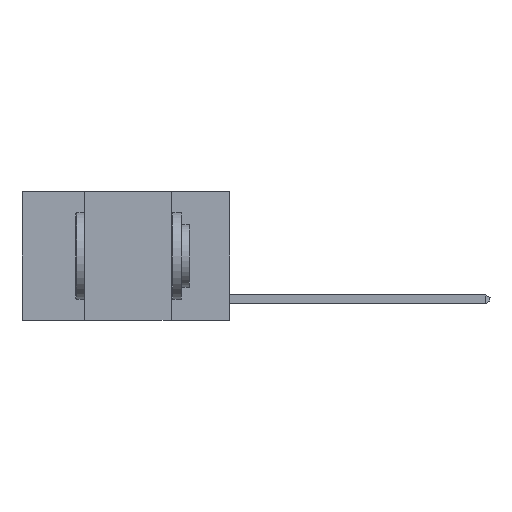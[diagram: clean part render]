
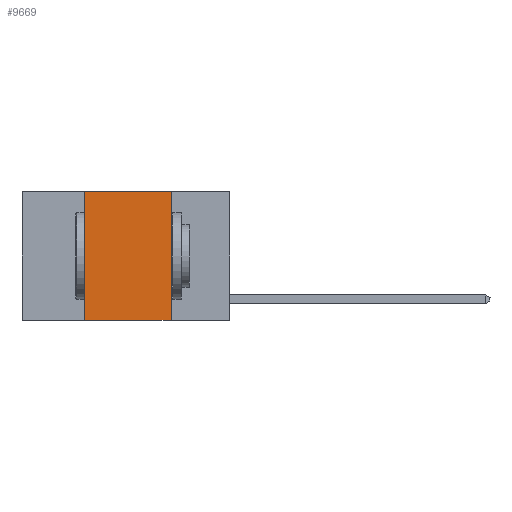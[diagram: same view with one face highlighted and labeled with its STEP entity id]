
A CAD part, left-side view. The second image highlights one B-rep face of the part: STEP entity #9669.
In plain terms, the highlighted planar face has unit normal (-1, 0, 0).
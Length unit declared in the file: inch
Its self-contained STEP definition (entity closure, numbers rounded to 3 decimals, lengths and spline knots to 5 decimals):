
#404 = VECTOR ( 'NONE', #17298, 39.37008 ) ;
#805 = VECTOR ( 'NONE', #9527, 39.37008 ) ;
#907 = VERTEX_POINT ( 'NONE', #20574 ) ;
#2370 = CARTESIAN_POINT ( 'NONE',  ( 0., 0.17, 0. ) ) ;
#3135 = ORIENTED_EDGE ( 'NONE', *, *, #13218, .F. ) ;
#3242 = ORIENTED_EDGE ( 'NONE', *, *, #9763, .F. ) ;
#3500 = EDGE_CURVE ( 'NONE', #18700, #907, #11289, .T. ) ;
#3995 = CARTESIAN_POINT ( 'NONE',  ( 0., 0.6, 0. ) ) ;
#5127 = LINE ( 'NONE', #18845, #20868 ) ;
#5535 = DIRECTION ( 'NONE',  ( 0., 0., -1. ) ) ;
#6553 = ORIENTED_EDGE ( 'NONE', *, *, #19326, .F. ) ;
#6944 = PLANE ( 'NONE',  #9436 ) ;
#7928 = EDGE_LOOP ( 'NONE', ( #6553, #3135, #3242, #18832 ) ) ;
#9130 = DIRECTION ( 'NONE',  ( 0., -1., 0. ) ) ;
#9436 = AXIS2_PLACEMENT_3D ( 'NONE', #3995, #13340, #5535 ) ;
#9504 = CARTESIAN_POINT ( 'NONE',  ( 0., 0.6, -0.37 ) ) ;
#9527 = DIRECTION ( 'NONE',  ( 0., 0., 1. ) ) ;
#9669 = ADVANCED_FACE ( 'NONE', ( #24513 ), #6944, .F. ) ;
#9763 = EDGE_CURVE ( 'NONE', #18700, #21294, #17203, .T. ) ;
#9905 = CARTESIAN_POINT ( 'NONE',  ( 0., 0.42, 0. ) ) ;
#10239 = DIRECTION ( 'NONE',  ( 0., 0., -1. ) ) ;
#11289 = LINE ( 'NONE', #9504, #404 ) ;
#13218 = EDGE_CURVE ( 'NONE', #21294, #23020, #5127, .T. ) ;
#13340 = DIRECTION ( 'NONE',  ( 1., 0., 0. ) ) ;
#13375 = CARTESIAN_POINT ( 'NONE',  ( 0., 0.42, 0. ) ) ;
#16499 = VECTOR ( 'NONE', #10239, 39.37008 ) ;
#17203 = LINE ( 'NONE', #9905, #805 ) ;
#17298 = DIRECTION ( 'NONE',  ( 0., -1., 0. ) ) ;
#17789 = LINE ( 'NONE', #2370, #16499 ) ;
#18700 = VERTEX_POINT ( 'NONE', #24403 ) ;
#18832 = ORIENTED_EDGE ( 'NONE', *, *, #3500, .T. ) ;
#18845 = CARTESIAN_POINT ( 'NONE',  ( 0., 0.6, 0. ) ) ;
#19326 = EDGE_CURVE ( 'NONE', #23020, #907, #17789, .T. ) ;
#20574 = CARTESIAN_POINT ( 'NONE',  ( 0., 0.17, -0.37 ) ) ;
#20868 = VECTOR ( 'NONE', #9130, 39.37008 ) ;
#21091 = CARTESIAN_POINT ( 'NONE',  ( 0., 0.17, 0. ) ) ;
#21294 = VERTEX_POINT ( 'NONE', #13375 ) ;
#23020 = VERTEX_POINT ( 'NONE', #21091 ) ;
#24403 = CARTESIAN_POINT ( 'NONE',  ( 0., 0.42, -0.37 ) ) ;
#24513 = FACE_OUTER_BOUND ( 'NONE', #7928, .T. ) ;
